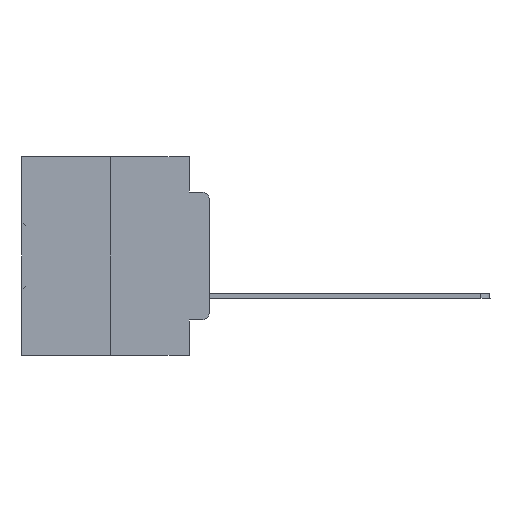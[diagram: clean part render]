
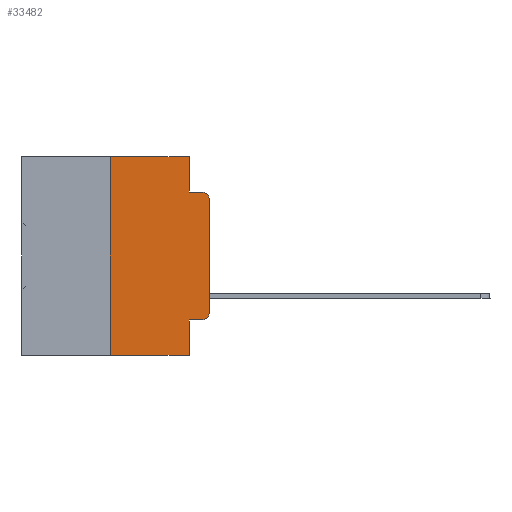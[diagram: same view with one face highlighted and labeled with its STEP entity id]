
A CAD part, left-side view. The second image highlights one B-rep face of the part: STEP entity #33482.
In plain terms, the highlighted planar face has unit normal (-1, 0, 0).
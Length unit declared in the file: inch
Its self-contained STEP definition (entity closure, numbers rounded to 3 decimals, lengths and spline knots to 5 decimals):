
#473 = CARTESIAN_POINT ( 'NONE',  ( 0., 0.473, -0.5 ) ) ;
#1049 = VERTEX_POINT ( 'NONE', #26833 ) ;
#1353 = LINE ( 'NONE', #27809, #23777 ) ;
#1746 = CARTESIAN_POINT ( 'NONE',  ( 0., 0.051, -0.0885 ) ) ;
#1876 = VERTEX_POINT ( 'NONE', #33640 ) ;
#2337 = EDGE_CURVE ( 'NONE', #1876, #1049, #23890, .T. ) ;
#2796 = CARTESIAN_POINT ( 'NONE',  ( 0., 0.051, -0.4115 ) ) ;
#3872 = CARTESIAN_POINT ( 'NONE',  ( 0., 0.051, -0.0885 ) ) ;
#4823 = CARTESIAN_POINT ( 'NONE',  ( 0., 0., -0.1085 ) ) ;
#4873 = ORIENTED_EDGE ( 'NONE', *, *, #20524, .F. ) ;
#5026 = LINE ( 'NONE', #473, #24435 ) ;
#5569 = CARTESIAN_POINT ( 'NONE',  ( 0., 0.02, -0.0885 ) ) ;
#6360 = ORIENTED_EDGE ( 'NONE', *, *, #30077, .F. ) ;
#6693 = CARTESIAN_POINT ( 'NONE',  ( 0., 0.02, -0.3915 ) ) ;
#6964 = VERTEX_POINT ( 'NONE', #20545 ) ;
#7213 = CARTESIAN_POINT ( 'NONE',  ( 0., 0.25, -0.5 ) ) ;
#7314 = ORIENTED_EDGE ( 'NONE', *, *, #26399, .T. ) ;
#7660 = ORIENTED_EDGE ( 'NONE', *, *, #33085, .T. ) ;
#8098 = VECTOR ( 'NONE', #11098, 39.37008 ) ;
#8202 = LINE ( 'NONE', #1746, #15414 ) ;
#8408 = ORIENTED_EDGE ( 'NONE', *, *, #16706, .T. ) ;
#8779 = CARTESIAN_POINT ( 'NONE',  ( 0., 0.25, 0. ) ) ;
#9101 = DIRECTION ( 'NONE',  ( 0., -1., 0. ) ) ;
#9408 = LINE ( 'NONE', #8779, #14490 ) ;
#10067 = FACE_OUTER_BOUND ( 'NONE', #23971, .T. ) ;
#10533 = ORIENTED_EDGE ( 'NONE', *, *, #11366, .F. ) ;
#10580 = VERTEX_POINT ( 'NONE', #7213 ) ;
#10910 = CIRCLE ( 'NONE', #25284, 0.02 ) ;
#10963 = CARTESIAN_POINT ( 'NONE',  ( 0., 0.051, 0. ) ) ;
#11098 = DIRECTION ( 'NONE',  ( 0., 0., 1. ) ) ;
#11366 = EDGE_CURVE ( 'NONE', #18001, #26059, #8202, .T. ) ;
#11511 = DIRECTION ( 'NONE',  ( 0., 0., 1. ) ) ;
#11666 = DIRECTION ( 'NONE',  ( -1., 0., 0. ) ) ;
#11980 = DIRECTION ( 'NONE',  ( 0., -1., 0. ) ) ;
#12194 = ORIENTED_EDGE ( 'NONE', *, *, #14154, .T. ) ;
#12330 = EDGE_CURVE ( 'NONE', #1876, #23679, #1353, .T. ) ;
#12345 = ORIENTED_EDGE ( 'NONE', *, *, #2337, .T. ) ;
#12644 = VERTEX_POINT ( 'NONE', #22411 ) ;
#12772 = AXIS2_PLACEMENT_3D ( 'NONE', #17262, #11666, #33235 ) ;
#13556 = CARTESIAN_POINT ( 'NONE',  ( 0., 0.051, -0.5 ) ) ;
#13681 = AXIS2_PLACEMENT_3D ( 'NONE', #24164, #29559, #32840 ) ;
#14154 = EDGE_CURVE ( 'NONE', #1049, #12644, #10910, .T. ) ;
#14165 = DIRECTION ( 'NONE',  ( 0., 0., -1. ) ) ;
#14481 = DIRECTION ( 'NONE',  ( -1., 0., 0. ) ) ;
#14490 = VECTOR ( 'NONE', #11511, 39.37008 ) ;
#15414 = VECTOR ( 'NONE', #31456, 39.37008 ) ;
#15853 = LINE ( 'NONE', #31528, #28488 ) ;
#16706 = EDGE_CURVE ( 'NONE', #10580, #23679, #5026, .T. ) ;
#17262 = CARTESIAN_POINT ( 'NONE',  ( 0., 0.02, -0.1085 ) ) ;
#18001 = VERTEX_POINT ( 'NONE', #3872 ) ;
#19538 = VERTEX_POINT ( 'NONE', #4823 ) ;
#20524 = EDGE_CURVE ( 'NONE', #20692, #18001, #28436, .T. ) ;
#20545 = CARTESIAN_POINT ( 'NONE',  ( 0., 0.25, 0. ) ) ;
#20692 = VERTEX_POINT ( 'NONE', #28333 ) ;
#21575 = PLANE ( 'NONE',  #13681 ) ;
#22411 = CARTESIAN_POINT ( 'NONE',  ( 0., 0., -0.3915 ) ) ;
#23679 = VERTEX_POINT ( 'NONE', #13556 ) ;
#23777 = VECTOR ( 'NONE', #14165, 39.37008 ) ;
#23890 = LINE ( 'NONE', #2796, #33570 ) ;
#23971 = EDGE_LOOP ( 'NONE', ( #7314, #7660, #10533, #4873, #25584, #6360, #8408, #30152, #12345, #12194 ) ) ;
#24164 = CARTESIAN_POINT ( 'NONE',  ( 0., 0.473, 0. ) ) ;
#24295 = DIRECTION ( 'NONE',  ( 0., 0., -1. ) ) ;
#24435 = VECTOR ( 'NONE', #9101, 39.37008 ) ;
#25110 = EDGE_CURVE ( 'NONE', #6964, #20692, #15853, .T. ) ;
#25284 = AXIS2_PLACEMENT_3D ( 'NONE', #6693, #14481, #25566 ) ;
#25566 = DIRECTION ( 'NONE',  ( 0., 0., -1. ) ) ;
#25584 = ORIENTED_EDGE ( 'NONE', *, *, #25110, .F. ) ;
#26059 = VERTEX_POINT ( 'NONE', #5569 ) ;
#26399 = EDGE_CURVE ( 'NONE', #12644, #19538, #32987, .T. ) ;
#26833 = CARTESIAN_POINT ( 'NONE',  ( 0., 0.02, -0.4115 ) ) ;
#26997 = CARTESIAN_POINT ( 'NONE',  ( 0., 0., 0. ) ) ;
#27809 = CARTESIAN_POINT ( 'NONE',  ( 0., 0.051, 0. ) ) ;
#28333 = CARTESIAN_POINT ( 'NONE',  ( 0., 0.051, 0. ) ) ;
#28436 = LINE ( 'NONE', #10963, #31361 ) ;
#28488 = VECTOR ( 'NONE', #11980, 39.37008 ) ;
#29559 = DIRECTION ( 'NONE',  ( 1., 0., 0. ) ) ;
#30077 = EDGE_CURVE ( 'NONE', #10580, #6964, #9408, .T. ) ;
#30152 = ORIENTED_EDGE ( 'NONE', *, *, #12330, .F. ) ;
#31361 = VECTOR ( 'NONE', #24295, 39.37008 ) ;
#31456 = DIRECTION ( 'NONE',  ( 0., -1., 0. ) ) ;
#31528 = CARTESIAN_POINT ( 'NONE',  ( 0., 0.473, 0. ) ) ;
#31984 = CIRCLE ( 'NONE', #12772, 0.02 ) ;
#32381 = DIRECTION ( 'NONE',  ( 0., -1., 0. ) ) ;
#32840 = DIRECTION ( 'NONE',  ( 0., 0., -1. ) ) ;
#32987 = LINE ( 'NONE', #26997, #8098 ) ;
#33085 = EDGE_CURVE ( 'NONE', #19538, #26059, #31984, .T. ) ;
#33235 = DIRECTION ( 'NONE',  ( 0., 0., -1. ) ) ;
#33482 = ADVANCED_FACE ( 'NONE', ( #10067 ), #21575, .F. ) ;
#33570 = VECTOR ( 'NONE', #32381, 39.37008 ) ;
#33640 = CARTESIAN_POINT ( 'NONE',  ( 0., 0.051, -0.4115 ) ) ;
